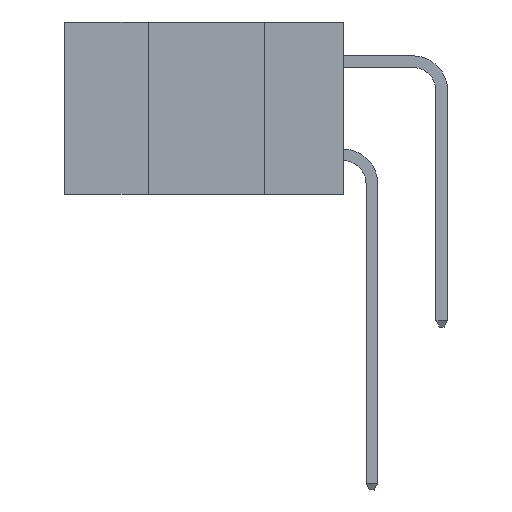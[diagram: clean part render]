
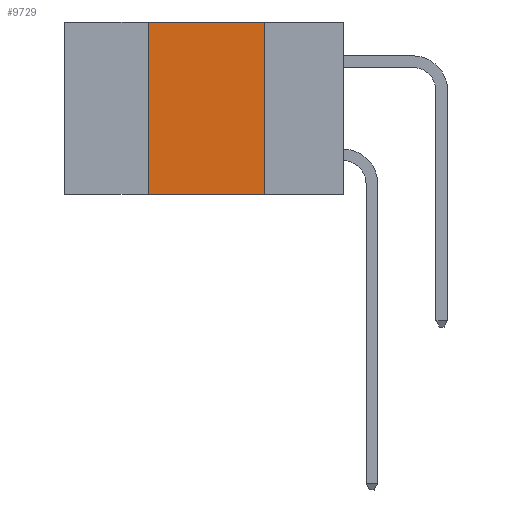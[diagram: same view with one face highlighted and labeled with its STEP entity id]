
A CAD part, left-side view. The second image highlights one B-rep face of the part: STEP entity #9729.
In plain terms, the highlighted planar face has unit normal (-1, 0, 0).
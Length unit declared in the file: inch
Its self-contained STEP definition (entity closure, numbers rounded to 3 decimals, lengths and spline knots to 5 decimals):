
#584 = DIRECTION ( 'NONE',  ( 0., 0., -1. ) ) ;
#1563 = EDGE_CURVE ( 'NONE', #17233, #23010, #20781, .T. ) ;
#2621 = VECTOR ( 'NONE', #16472, 39.37008 ) ;
#2897 = EDGE_LOOP ( 'NONE', ( #9828, #9736, #11444, #22370 ) ) ;
#3105 = DIRECTION ( 'NONE',  ( 0., -1., 0. ) ) ;
#6924 = DIRECTION ( 'NONE',  ( 1., 0., 0. ) ) ;
#7331 = CARTESIAN_POINT ( 'NONE',  ( 0., 0.42, -0.37 ) ) ;
#8058 = VECTOR ( 'NONE', #3105, 39.37008 ) ;
#8227 = EDGE_CURVE ( 'NONE', #17233, #10831, #11711, .T. ) ;
#9656 = VERTEX_POINT ( 'NONE', #17927 ) ;
#9729 = ADVANCED_FACE ( 'NONE', ( #12454 ), #19652, .F. ) ;
#9736 = ORIENTED_EDGE ( 'NONE', *, *, #20314, .F. ) ;
#9828 = ORIENTED_EDGE ( 'NONE', *, *, #17687, .F. ) ;
#10601 = LINE ( 'NONE', #19718, #17307 ) ;
#10831 = VERTEX_POINT ( 'NONE', #20290 ) ;
#11444 = ORIENTED_EDGE ( 'NONE', *, *, #8227, .F. ) ;
#11711 = LINE ( 'NONE', #14667, #2621 ) ;
#12236 = CARTESIAN_POINT ( 'NONE',  ( 0., 0.6, 0. ) ) ;
#12386 = CARTESIAN_POINT ( 'NONE',  ( 0., 0.17, -0.37 ) ) ;
#12454 = FACE_OUTER_BOUND ( 'NONE', #2897, .T. ) ;
#12704 = VECTOR ( 'NONE', #584, 39.37008 ) ;
#14020 = DIRECTION ( 'NONE',  ( 0., 0., -1. ) ) ;
#14667 = CARTESIAN_POINT ( 'NONE',  ( 0., 0.42, 0. ) ) ;
#14843 = CARTESIAN_POINT ( 'NONE',  ( 0., 0.17, 0. ) ) ;
#16472 = DIRECTION ( 'NONE',  ( 0., 0., 1. ) ) ;
#17233 = VERTEX_POINT ( 'NONE', #7331 ) ;
#17307 = VECTOR ( 'NONE', #21642, 39.37008 ) ;
#17687 = EDGE_CURVE ( 'NONE', #9656, #23010, #20624, .T. ) ;
#17927 = CARTESIAN_POINT ( 'NONE',  ( 0., 0.17, 0. ) ) ;
#19308 = CARTESIAN_POINT ( 'NONE',  ( 0., 0.6, -0.37 ) ) ;
#19652 = PLANE ( 'NONE',  #20393 ) ;
#19718 = CARTESIAN_POINT ( 'NONE',  ( 0., 0.6, 0. ) ) ;
#20290 = CARTESIAN_POINT ( 'NONE',  ( 0., 0.42, 0. ) ) ;
#20314 = EDGE_CURVE ( 'NONE', #10831, #9656, #10601, .T. ) ;
#20393 = AXIS2_PLACEMENT_3D ( 'NONE', #12236, #6924, #14020 ) ;
#20624 = LINE ( 'NONE', #14843, #12704 ) ;
#20781 = LINE ( 'NONE', #19308, #8058 ) ;
#21642 = DIRECTION ( 'NONE',  ( 0., -1., 0. ) ) ;
#22370 = ORIENTED_EDGE ( 'NONE', *, *, #1563, .T. ) ;
#23010 = VERTEX_POINT ( 'NONE', #12386 ) ;
